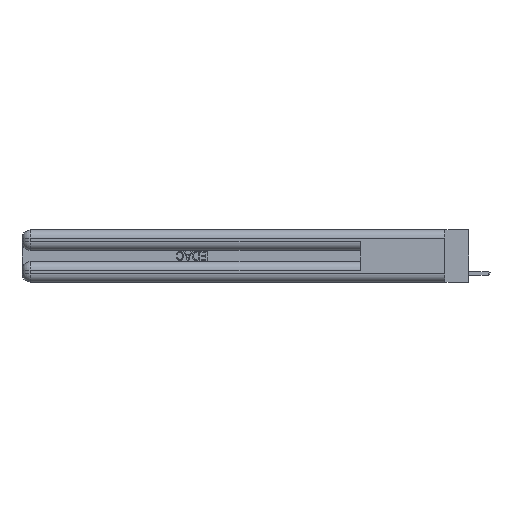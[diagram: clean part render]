
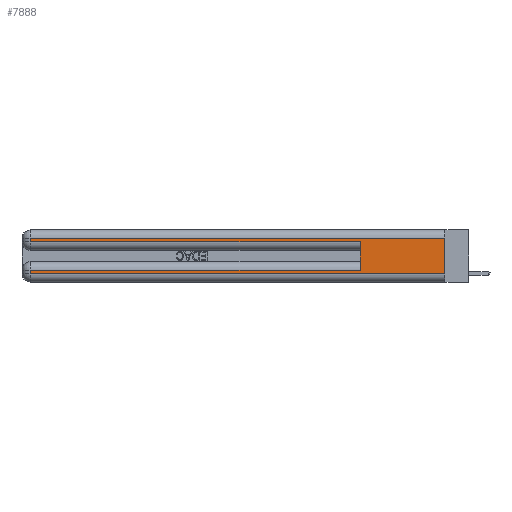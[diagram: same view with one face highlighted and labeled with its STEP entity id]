
A CAD part, left-side view. The second image highlights one B-rep face of the part: STEP entity #7888.
In plain terms, the highlighted planar face has unit normal (-1, 0, 0).
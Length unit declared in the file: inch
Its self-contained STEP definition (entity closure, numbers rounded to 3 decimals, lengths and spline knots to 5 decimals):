
#86 = CARTESIAN_POINT ( 'NONE',  ( 0., 0., 0.31 ) ) ;
#119 = ORIENTED_EDGE ( 'NONE', *, *, #20932, .T. ) ;
#1433 = DIRECTION ( 'NONE',  ( 0., 0., -1. ) ) ;
#1690 = LINE ( 'NONE', #22804, #11679 ) ;
#1739 = CARTESIAN_POINT ( 'NONE',  ( 0., 2.94, 0.285 ) ) ;
#1757 = EDGE_CURVE ( 'NONE', #16369, #3844, #15079, .T. ) ;
#2136 = VERTEX_POINT ( 'NONE', #6576 ) ;
#3290 = ORIENTED_EDGE ( 'NONE', *, *, #11364, .F. ) ;
#3469 = LINE ( 'NONE', #19001, #14487 ) ;
#3844 = VERTEX_POINT ( 'NONE', #27207 ) ;
#4509 = LINE ( 'NONE', #16040, #26133 ) ;
#4603 = CARTESIAN_POINT ( 'NONE',  ( 0., 2.94, 0.37 ) ) ;
#4688 = EDGE_CURVE ( 'NONE', #3844, #21594, #21465, .T. ) ;
#5187 = VERTEX_POINT ( 'NONE', #11461 ) ;
#5612 = CARTESIAN_POINT ( 'NONE',  ( 0., 0., 0.085 ) ) ;
#5943 = DIRECTION ( 'NONE',  ( 1., 0., 0. ) ) ;
#6147 = ORIENTED_EDGE ( 'NONE', *, *, #6268, .T. ) ;
#6268 = EDGE_CURVE ( 'NONE', #2136, #24983, #22765, .T. ) ;
#6311 = DIRECTION ( 'NONE',  ( 0., 1., 0. ) ) ;
#6576 = CARTESIAN_POINT ( 'NONE',  ( 0., 2.94, 0.085 ) ) ;
#6716 = DIRECTION ( 'NONE',  ( 0., 0., -1. ) ) ;
#7431 = ORIENTED_EDGE ( 'NONE', *, *, #7699, .T. ) ;
#7467 = VECTOR ( 'NONE', #26600, 39.37008 ) ;
#7533 = DIRECTION ( 'NONE',  ( 0., -1., 0. ) ) ;
#7541 = VERTEX_POINT ( 'NONE', #9198 ) ;
#7699 = EDGE_CURVE ( 'NONE', #24983, #7541, #1690, .T. ) ;
#7888 = ADVANCED_FACE ( 'NONE', ( #13350 ), #10316, .F. ) ;
#8649 = VERTEX_POINT ( 'NONE', #23157 ) ;
#9114 = VECTOR ( 'NONE', #6311, 39.37008 ) ;
#9198 = CARTESIAN_POINT ( 'NONE',  ( 0., 0., 0.06 ) ) ;
#9371 = VECTOR ( 'NONE', #19175, 39.37008 ) ;
#9671 = EDGE_CURVE ( 'NONE', #8649, #2136, #15573, .T. ) ;
#10316 = PLANE ( 'NONE',  #21398 ) ;
#10988 = CARTESIAN_POINT ( 'NONE',  ( 0., 0., 0.31 ) ) ;
#11364 = EDGE_CURVE ( 'NONE', #8649, #5187, #3469, .T. ) ;
#11461 = CARTESIAN_POINT ( 'NONE',  ( 0., 0.6, 0.285 ) ) ;
#11679 = VECTOR ( 'NONE', #22622, 39.37008 ) ;
#12166 = CARTESIAN_POINT ( 'NONE',  ( 0., 0., 0.37 ) ) ;
#12320 = ORIENTED_EDGE ( 'NONE', *, *, #1757, .T. ) ;
#13080 = LINE ( 'NONE', #12166, #22087 ) ;
#13350 = FACE_OUTER_BOUND ( 'NONE', #14211, .T. ) ;
#14211 = EDGE_LOOP ( 'NONE', ( #25873, #12320, #21933, #119, #3290, #23128, #6147, #7431 ) ) ;
#14487 = VECTOR ( 'NONE', #21219, 39.37008 ) ;
#15079 = LINE ( 'NONE', #86, #9371 ) ;
#15573 = LINE ( 'NONE', #5612, #9114 ) ;
#16040 = CARTESIAN_POINT ( 'NONE',  ( 0., 0., 0.285 ) ) ;
#16369 = VERTEX_POINT ( 'NONE', #10988 ) ;
#16495 = DIRECTION ( 'NONE',  ( 0., 0., -1. ) ) ;
#16549 = EDGE_CURVE ( 'NONE', #16369, #7541, #13080, .T. ) ;
#18345 = CARTESIAN_POINT ( 'NONE',  ( 0., 2.94, 0.37 ) ) ;
#19001 = CARTESIAN_POINT ( 'NONE',  ( 0., 0.6, 0.145 ) ) ;
#19011 = CARTESIAN_POINT ( 'NONE',  ( 0., 2.94, 0.06 ) ) ;
#19110 = VECTOR ( 'NONE', #6716, 39.37008 ) ;
#19175 = DIRECTION ( 'NONE',  ( 0., 1., 0. ) ) ;
#20745 = CARTESIAN_POINT ( 'NONE',  ( 0., 0., 0.37 ) ) ;
#20932 = EDGE_CURVE ( 'NONE', #21594, #5187, #4509, .T. ) ;
#21219 = DIRECTION ( 'NONE',  ( 0., 0., 1. ) ) ;
#21398 = AXIS2_PLACEMENT_3D ( 'NONE', #20745, #5943, #16495 ) ;
#21465 = LINE ( 'NONE', #18345, #7467 ) ;
#21594 = VERTEX_POINT ( 'NONE', #1739 ) ;
#21933 = ORIENTED_EDGE ( 'NONE', *, *, #4688, .T. ) ;
#22087 = VECTOR ( 'NONE', #1433, 39.37008 ) ;
#22622 = DIRECTION ( 'NONE',  ( 0., -1., 0. ) ) ;
#22765 = LINE ( 'NONE', #4603, #19110 ) ;
#22804 = CARTESIAN_POINT ( 'NONE',  ( 0., 0., 0.06 ) ) ;
#23128 = ORIENTED_EDGE ( 'NONE', *, *, #9671, .T. ) ;
#23157 = CARTESIAN_POINT ( 'NONE',  ( 0., 0.6, 0.085 ) ) ;
#24983 = VERTEX_POINT ( 'NONE', #19011 ) ;
#25873 = ORIENTED_EDGE ( 'NONE', *, *, #16549, .F. ) ;
#26133 = VECTOR ( 'NONE', #7533, 39.37008 ) ;
#26600 = DIRECTION ( 'NONE',  ( 0., 0., -1. ) ) ;
#27207 = CARTESIAN_POINT ( 'NONE',  ( 0., 2.94, 0.31 ) ) ;
